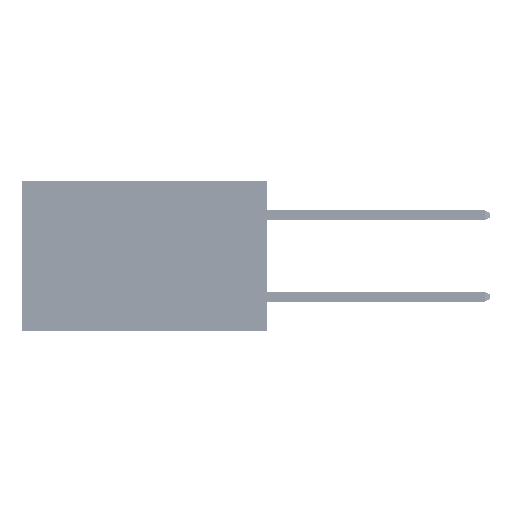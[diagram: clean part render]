
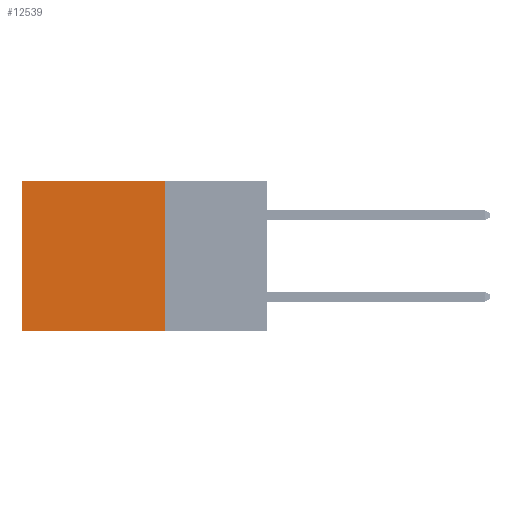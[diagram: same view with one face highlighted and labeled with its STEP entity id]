
A CAD part, left-side view. The second image highlights one B-rep face of the part: STEP entity #12539.
In plain terms, the highlighted planar face has unit normal (-1, 0, 0).
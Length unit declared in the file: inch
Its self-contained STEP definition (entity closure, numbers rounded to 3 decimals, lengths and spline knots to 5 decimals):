
#385 = VECTOR ( 'NONE', #24791, 39.37008 ) ;
#1524 = VERTEX_POINT ( 'NONE', #15259 ) ;
#1691 = CARTESIAN_POINT ( 'NONE',  ( 0.2875, 0.6, 0. ) ) ;
#2547 = LINE ( 'NONE', #27135, #41054 ) ;
#4644 = CARTESIAN_POINT ( 'NONE',  ( 0.2875, 0.25, 0. ) ) ;
#6603 = VERTEX_POINT ( 'NONE', #14836 ) ;
#7078 = VERTEX_POINT ( 'NONE', #24117 ) ;
#7247 = DIRECTION ( 'NONE',  ( 0., 1., 0. ) ) ;
#7377 = DIRECTION ( 'NONE',  ( 0., 1., 0. ) ) ;
#7780 = ORIENTED_EDGE ( 'NONE', *, *, #16301, .T. ) ;
#8231 = CARTESIAN_POINT ( 'NONE',  ( 0.2875, 0.6, 0. ) ) ;
#9189 = DIRECTION ( 'NONE',  ( 0., 0., -1. ) ) ;
#10688 = CARTESIAN_POINT ( 'NONE',  ( 0.2875, 0.25, 0. ) ) ;
#12539 = ADVANCED_FACE ( 'NONE', ( #45815 ), #45030, .F. ) ;
#12849 = ORIENTED_EDGE ( 'NONE', *, *, #29489, .T. ) ;
#14836 = CARTESIAN_POINT ( 'NONE',  ( 0.2875, 0.6, -0.37 ) ) ;
#15259 = CARTESIAN_POINT ( 'NONE',  ( 0.2875, 0.25, 0. ) ) ;
#16301 = EDGE_CURVE ( 'NONE', #1524, #38715, #2547, .T. ) ;
#17645 = DIRECTION ( 'NONE',  ( 0., 0., -1. ) ) ;
#22318 = LINE ( 'NONE', #46350, #25510 ) ;
#23155 = ORIENTED_EDGE ( 'NONE', *, *, #50829, .F. ) ;
#24117 = CARTESIAN_POINT ( 'NONE',  ( 0.2875, 0.25, -0.37 ) ) ;
#24791 = DIRECTION ( 'NONE',  ( 0., 0., -1. ) ) ;
#25510 = VECTOR ( 'NONE', #7377, 39.37008 ) ;
#27135 = CARTESIAN_POINT ( 'NONE',  ( 0.2875, 0.25, 0. ) ) ;
#29489 = EDGE_CURVE ( 'NONE', #38715, #6603, #29686, .T. ) ;
#29686 = LINE ( 'NONE', #1691, #31676 ) ;
#31676 = VECTOR ( 'NONE', #17645, 39.37008 ) ;
#31830 = EDGE_LOOP ( 'NONE', ( #12849, #23155, #47324, #7780 ) ) ;
#38715 = VERTEX_POINT ( 'NONE', #8231 ) ;
#40443 = LINE ( 'NONE', #4644, #385 ) ;
#40669 = AXIS2_PLACEMENT_3D ( 'NONE', #10688, #46773, #9189 ) ;
#41054 = VECTOR ( 'NONE', #7247, 39.37008 ) ;
#41505 = EDGE_CURVE ( 'NONE', #1524, #7078, #40443, .T. ) ;
#45030 = PLANE ( 'NONE',  #40669 ) ;
#45815 = FACE_OUTER_BOUND ( 'NONE', #31830, .T. ) ;
#46350 = CARTESIAN_POINT ( 'NONE',  ( 0.2875, 0.25, -0.37 ) ) ;
#46773 = DIRECTION ( 'NONE',  ( 1., 0., 0. ) ) ;
#47324 = ORIENTED_EDGE ( 'NONE', *, *, #41505, .F. ) ;
#50829 = EDGE_CURVE ( 'NONE', #7078, #6603, #22318, .T. ) ;
